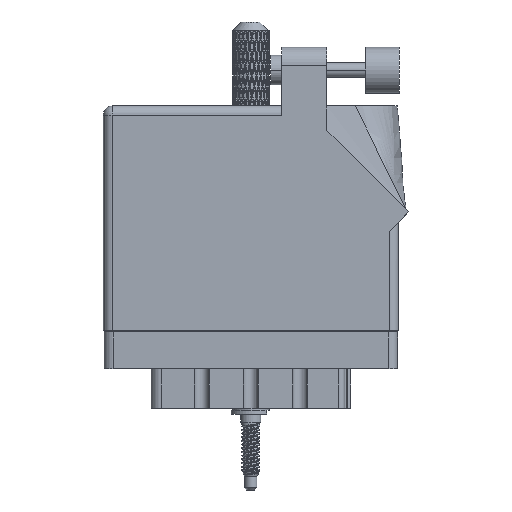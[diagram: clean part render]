
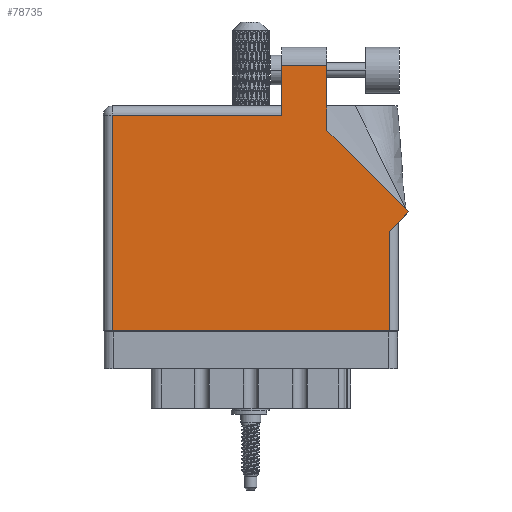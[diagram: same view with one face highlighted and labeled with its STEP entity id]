
A CAD part, front view. The second image highlights one B-rep face of the part: STEP entity #78735.
In plain terms, the highlighted face is planar.
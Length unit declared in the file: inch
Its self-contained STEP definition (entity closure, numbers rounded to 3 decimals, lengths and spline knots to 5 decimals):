
#4632 = CARTESIAN_POINT ( 'NONE',  ( 1.948, 0.737, 0. ) ) ;
#4844 = VERTEX_POINT ( 'NONE', #48132 ) ;
#7773 = VECTOR ( 'NONE', #87951, 39.37008 ) ;
#8290 = CARTESIAN_POINT ( 'NONE',  ( 0., 1.53, 0. ) ) ;
#8612 = LINE ( 'NONE', #41679, #98762 ) ;
#9060 = VERTEX_POINT ( 'NONE', #94541 ) ;
#10676 = ORIENTED_EDGE ( 'NONE', *, *, #88865, .T. ) ;
#11161 = CARTESIAN_POINT ( 'NONE',  ( 0.062, 0., 0. ) ) ;
#13140 = CARTESIAN_POINT ( 'NONE',  ( 0.062, 0., 0. ) ) ;
#14525 = CARTESIAN_POINT ( 'NONE',  ( 1.948, 0., 0. ) ) ;
#15682 = VERTEX_POINT ( 'NONE', #13140 ) ;
#17995 = CARTESIAN_POINT ( 'NONE',  ( 1.217, 1.53, 0. ) ) ;
#21926 = DIRECTION ( 'NONE',  ( 0., 1., 0. ) ) ;
#24105 = DIRECTION ( 'NONE',  ( -1., 0., 0. ) ) ;
#25581 = LINE ( 'NONE', #17995, #57977 ) ;
#25684 = VERTEX_POINT ( 'NONE', #74478 ) ;
#27334 = VERTEX_POINT ( 'NONE', #14525 ) ;
#27480 = VECTOR ( 'NONE', #77806, 39.37008 ) ;
#28308 = EDGE_CURVE ( 'NONE', #4844, #84989, #36678, .T. ) ;
#29388 = VECTOR ( 'NONE', #55121, 39.37008 ) ;
#30492 = FACE_OUTER_BOUND ( 'NONE', #54558, .T. ) ;
#35435 = ORIENTED_EDGE ( 'NONE', *, *, #84815, .T. ) ;
#36532 = ORIENTED_EDGE ( 'NONE', *, *, #72776, .T. ) ;
#36678 = LINE ( 'NONE', #44835, #27480 ) ;
#37552 = LINE ( 'NONE', #11161, #41072 ) ;
#38851 = LINE ( 'NONE', #87019, #29388 ) ;
#41072 = VECTOR ( 'NONE', #52368, 39.37008 ) ;
#41679 = CARTESIAN_POINT ( 'NONE',  ( 1.524, 1.36442, 0. ) ) ;
#44835 = CARTESIAN_POINT ( 'NONE',  ( 2.08071, 0.80771, 0. ) ) ;
#48132 = CARTESIAN_POINT ( 'NONE',  ( 2.08071, 0.80771, 0. ) ) ;
#48905 = CARTESIAN_POINT ( 'NONE',  ( 0.062, 1.468, 0. ) ) ;
#49450 = ORIENTED_EDGE ( 'NONE', *, *, #94431, .T. ) ;
#50479 = CARTESIAN_POINT ( 'NONE',  ( 1.217, 1.468, 0. ) ) ;
#50899 = ORIENTED_EDGE ( 'NONE', *, *, #104525, .T. ) ;
#51061 = DIRECTION ( 'NONE',  ( 0., -1., 0. ) ) ;
#52083 = VERTEX_POINT ( 'NONE', #83240 ) ;
#52368 = DIRECTION ( 'NONE',  ( 0., -1., 0. ) ) ;
#54558 = EDGE_LOOP ( 'NONE', ( #50899, #57350, #10676, #49450, #104210, #69475, #36532, #35435, #63804 ) ) ;
#54860 = VECTOR ( 'NONE', #92923, 39.37008 ) ;
#55008 = LINE ( 'NONE', #4632, #64170 ) ;
#55121 = DIRECTION ( 'NONE',  ( 1., 0., 0. ) ) ;
#55918 = EDGE_CURVE ( 'NONE', #25684, #9060, #60499, .T. ) ;
#57060 = EDGE_CURVE ( 'NONE', #64066, #15682, #37552, .T. ) ;
#57350 = ORIENTED_EDGE ( 'NONE', *, *, #55918, .T. ) ;
#57977 = VECTOR ( 'NONE', #51061, 39.37008 ) ;
#60110 = DIRECTION ( 'NONE',  ( 0., 1., 0. ) ) ;
#60257 = VERTEX_POINT ( 'NONE', #50479 ) ;
#60499 = LINE ( 'NONE', #101033, #54860 ) ;
#62706 = AXIS2_PLACEMENT_3D ( 'NONE', #8290, #89528, #88456 ) ;
#63804 = ORIENTED_EDGE ( 'NONE', *, *, #28308, .T. ) ;
#64066 = VERTEX_POINT ( 'NONE', #48905 ) ;
#64145 = CARTESIAN_POINT ( 'NONE',  ( 2.01, 0.737, 0. ) ) ;
#64170 = VECTOR ( 'NONE', #21926, 39.37008 ) ;
#69475 = ORIENTED_EDGE ( 'NONE', *, *, #102406, .T. ) ;
#72776 = EDGE_CURVE ( 'NONE', #27334, #52083, #55008, .T. ) ;
#74478 = CARTESIAN_POINT ( 'NONE',  ( 1.524, 1.805, 0. ) ) ;
#77806 = DIRECTION ( 'NONE',  ( -0.707, 0.707, 0. ) ) ;
#78735 = ADVANCED_FACE ( 'NONE', ( #30492 ), #90587, .F. ) ;
#82558 = CARTESIAN_POINT ( 'NONE',  ( 0., 1.468, 0. ) ) ;
#83240 = CARTESIAN_POINT ( 'NONE',  ( 1.948, 0.675, 0. ) ) ;
#84815 = EDGE_CURVE ( 'NONE', #52083, #4844, #89014, .T. ) ;
#84989 = VERTEX_POINT ( 'NONE', #86088 ) ;
#86088 = CARTESIAN_POINT ( 'NONE',  ( 1.524, 1.36442, 0. ) ) ;
#87019 = CARTESIAN_POINT ( 'NONE',  ( 0., 0., 0. ) ) ;
#87951 = DIRECTION ( 'NONE',  ( 0.707, 0.707, 0. ) ) ;
#88456 = DIRECTION ( 'NONE',  ( -1., 0., 0. ) ) ;
#88865 = EDGE_CURVE ( 'NONE', #9060, #60257, #25581, .T. ) ;
#89014 = LINE ( 'NONE', #64145, #7773 ) ;
#89528 = DIRECTION ( 'NONE',  ( 0., 0., -1. ) ) ;
#89723 = VECTOR ( 'NONE', #24105, 39.37008 ) ;
#90587 = PLANE ( 'NONE',  #62706 ) ;
#92923 = DIRECTION ( 'NONE',  ( -1., 0., 0. ) ) ;
#94431 = EDGE_CURVE ( 'NONE', #60257, #64066, #106393, .T. ) ;
#94541 = CARTESIAN_POINT ( 'NONE',  ( 1.217, 1.805, 0. ) ) ;
#98762 = VECTOR ( 'NONE', #60110, 39.37008 ) ;
#101033 = CARTESIAN_POINT ( 'NONE',  ( 1.217, 1.805, 0. ) ) ;
#102406 = EDGE_CURVE ( 'NONE', #15682, #27334, #38851, .T. ) ;
#104210 = ORIENTED_EDGE ( 'NONE', *, *, #57060, .T. ) ;
#104525 = EDGE_CURVE ( 'NONE', #84989, #25684, #8612, .T. ) ;
#106393 = LINE ( 'NONE', #82558, #89723 ) ;
